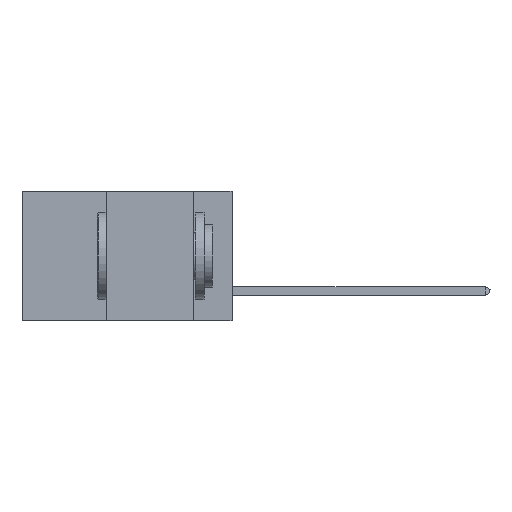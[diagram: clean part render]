
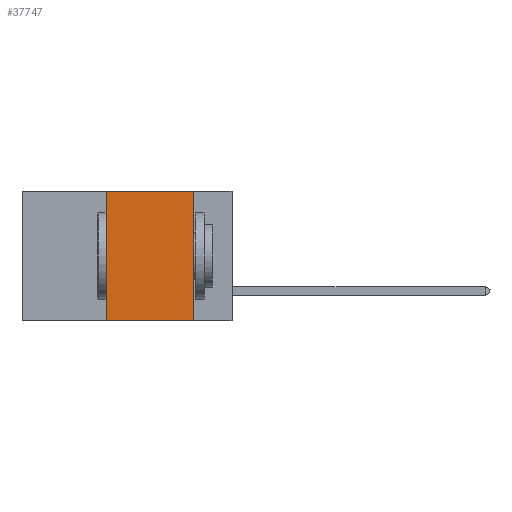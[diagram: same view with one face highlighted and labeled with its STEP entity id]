
A CAD part, left-side view. The second image highlights one B-rep face of the part: STEP entity #37747.
In plain terms, the highlighted planar face has unit normal (-1, 0, 0).
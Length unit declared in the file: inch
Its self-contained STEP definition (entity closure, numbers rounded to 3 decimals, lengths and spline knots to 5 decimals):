
#938 = DIRECTION ( 'NONE',  ( 1., 0., 0. ) ) ;
#2016 = CARTESIAN_POINT ( 'NONE',  ( 0., 0.11, 0. ) ) ;
#3995 = LINE ( 'NONE', #13601, #42800 ) ;
#5188 = CARTESIAN_POINT ( 'NONE',  ( 0., 0.6, 0. ) ) ;
#6023 = CARTESIAN_POINT ( 'NONE',  ( 0., 0.36, 0. ) ) ;
#6348 = ORIENTED_EDGE ( 'NONE', *, *, #16729, .F. ) ;
#6464 = LINE ( 'NONE', #13196, #44133 ) ;
#6640 = EDGE_CURVE ( 'NONE', #27383, #28202, #3995, .T. ) ;
#8631 = VECTOR ( 'NONE', #17465, 39.37008 ) ;
#8844 = CARTESIAN_POINT ( 'NONE',  ( 0., 0.11, -0.37 ) ) ;
#9867 = DIRECTION ( 'NONE',  ( 0., -1., 0. ) ) ;
#13196 = CARTESIAN_POINT ( 'NONE',  ( 0., 0.6, -0.37 ) ) ;
#13601 = CARTESIAN_POINT ( 'NONE',  ( 0., 0.6, 0. ) ) ;
#16729 = EDGE_CURVE ( 'NONE', #28202, #28561, #25576, .T. ) ;
#17465 = DIRECTION ( 'NONE',  ( 0., 0., -1. ) ) ;
#18224 = DIRECTION ( 'NONE',  ( 0., -1., 0. ) ) ;
#21379 = EDGE_CURVE ( 'NONE', #21827, #27383, #45502, .T. ) ;
#21827 = VERTEX_POINT ( 'NONE', #29394 ) ;
#22335 = CARTESIAN_POINT ( 'NONE',  ( 0., 0.11, 0. ) ) ;
#22844 = VECTOR ( 'NONE', #40167, 39.37008 ) ;
#25576 = LINE ( 'NONE', #2016, #8631 ) ;
#26377 = ORIENTED_EDGE ( 'NONE', *, *, #35843, .T. ) ;
#27383 = VERTEX_POINT ( 'NONE', #6023 ) ;
#28202 = VERTEX_POINT ( 'NONE', #22335 ) ;
#28561 = VERTEX_POINT ( 'NONE', #8844 ) ;
#29394 = CARTESIAN_POINT ( 'NONE',  ( 0., 0.36, -0.37 ) ) ;
#34469 = ORIENTED_EDGE ( 'NONE', *, *, #21379, .F. ) ;
#35659 = EDGE_LOOP ( 'NONE', ( #6348, #37384, #34469, #26377 ) ) ;
#35843 = EDGE_CURVE ( 'NONE', #21827, #28561, #6464, .T. ) ;
#37384 = ORIENTED_EDGE ( 'NONE', *, *, #6640, .F. ) ;
#37747 = ADVANCED_FACE ( 'NONE', ( #45778 ), #39256, .F. ) ;
#39256 = PLANE ( 'NONE',  #40750 ) ;
#40167 = DIRECTION ( 'NONE',  ( 0., 0., 1. ) ) ;
#40750 = AXIS2_PLACEMENT_3D ( 'NONE', #5188, #938, #47149 ) ;
#42651 = CARTESIAN_POINT ( 'NONE',  ( 0., 0.36, 0. ) ) ;
#42800 = VECTOR ( 'NONE', #18224, 39.37008 ) ;
#44133 = VECTOR ( 'NONE', #9867, 39.37008 ) ;
#45502 = LINE ( 'NONE', #42651, #22844 ) ;
#45778 = FACE_OUTER_BOUND ( 'NONE', #35659, .T. ) ;
#47149 = DIRECTION ( 'NONE',  ( 0., 0., -1. ) ) ;
